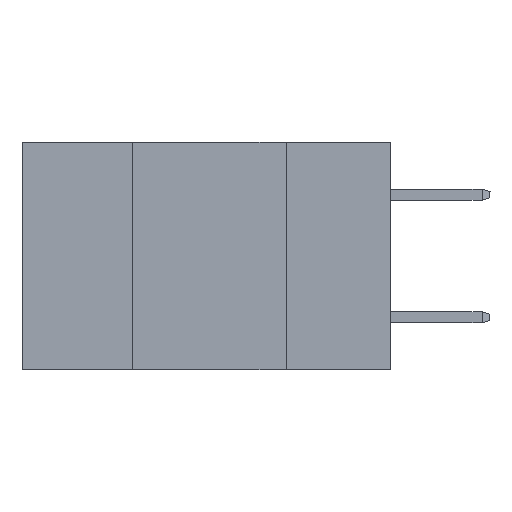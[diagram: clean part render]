
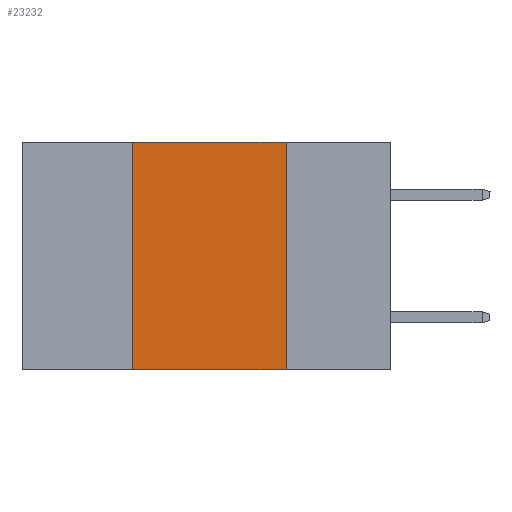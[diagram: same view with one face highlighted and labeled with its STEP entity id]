
A CAD part, left-side view. The second image highlights one B-rep face of the part: STEP entity #23232.
In plain terms, the highlighted planar face has unit normal (-1, 0, 0).
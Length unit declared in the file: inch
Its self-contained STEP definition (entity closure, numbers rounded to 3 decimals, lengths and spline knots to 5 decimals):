
#1600 = LINE ( 'NONE', #9367, #20444 ) ;
#1652 = VERTEX_POINT ( 'NONE', #19639 ) ;
#2672 = EDGE_LOOP ( 'NONE', ( #4461, #18030, #13629, #15254 ) ) ;
#4461 = ORIENTED_EDGE ( 'NONE', *, *, #9107, .F. ) ;
#5200 = LINE ( 'NONE', #16782, #27009 ) ;
#6072 = CARTESIAN_POINT ( 'NONE',  ( 0., 0.17, -0.37 ) ) ;
#6266 = VERTEX_POINT ( 'NONE', #21028 ) ;
#7134 = CARTESIAN_POINT ( 'NONE',  ( 0., 0.6, -0.37 ) ) ;
#9107 = EDGE_CURVE ( 'NONE', #6266, #26774, #1600, .T. ) ;
#9367 = CARTESIAN_POINT ( 'NONE',  ( 0., 0.17, 0. ) ) ;
#9639 = VECTOR ( 'NONE', #16969, 39.37008 ) ;
#10945 = DIRECTION ( 'NONE',  ( 0., 0., -1. ) ) ;
#11921 = DIRECTION ( 'NONE',  ( 0., -1., 0. ) ) ;
#12864 = LINE ( 'NONE', #7134, #25762 ) ;
#13347 = PLANE ( 'NONE',  #26280 ) ;
#13629 = ORIENTED_EDGE ( 'NONE', *, *, #26855, .F. ) ;
#15040 = EDGE_CURVE ( 'NONE', #1652, #26774, #12864, .T. ) ;
#15254 = ORIENTED_EDGE ( 'NONE', *, *, #15040, .T. ) ;
#16146 = FACE_OUTER_BOUND ( 'NONE', #2672, .T. ) ;
#16782 = CARTESIAN_POINT ( 'NONE',  ( 0., 0.6, 0. ) ) ;
#16969 = DIRECTION ( 'NONE',  ( 0., 0., 1. ) ) ;
#17628 = DIRECTION ( 'NONE',  ( 1., 0., 0. ) ) ;
#18030 = ORIENTED_EDGE ( 'NONE', *, *, #23629, .F. ) ;
#19364 = CARTESIAN_POINT ( 'NONE',  ( 0., 0.6, 0. ) ) ;
#19636 = DIRECTION ( 'NONE',  ( 0., 0., -1. ) ) ;
#19639 = CARTESIAN_POINT ( 'NONE',  ( 0., 0.42, -0.37 ) ) ;
#19737 = VERTEX_POINT ( 'NONE', #20407 ) ;
#20407 = CARTESIAN_POINT ( 'NONE',  ( 0., 0.42, 0. ) ) ;
#20444 = VECTOR ( 'NONE', #19636, 39.37008 ) ;
#21028 = CARTESIAN_POINT ( 'NONE',  ( 0., 0.17, 0. ) ) ;
#22870 = DIRECTION ( 'NONE',  ( 0., -1., 0. ) ) ;
#23232 = ADVANCED_FACE ( 'NONE', ( #16146 ), #13347, .F. ) ;
#23629 = EDGE_CURVE ( 'NONE', #19737, #6266, #5200, .T. ) ;
#25247 = CARTESIAN_POINT ( 'NONE',  ( 0., 0.42, 0. ) ) ;
#25762 = VECTOR ( 'NONE', #11921, 39.37008 ) ;
#26280 = AXIS2_PLACEMENT_3D ( 'NONE', #19364, #17628, #10945 ) ;
#26504 = LINE ( 'NONE', #25247, #9639 ) ;
#26774 = VERTEX_POINT ( 'NONE', #6072 ) ;
#26855 = EDGE_CURVE ( 'NONE', #1652, #19737, #26504, .T. ) ;
#27009 = VECTOR ( 'NONE', #22870, 39.37008 ) ;
